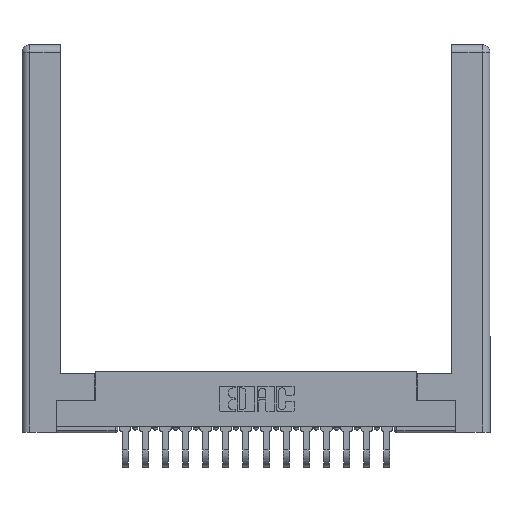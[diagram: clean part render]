
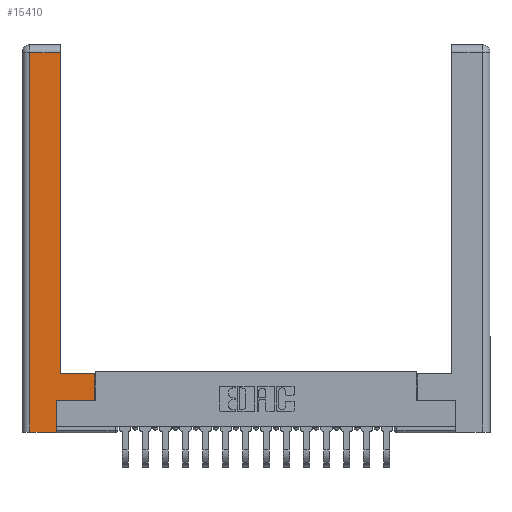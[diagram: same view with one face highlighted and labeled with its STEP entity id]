
A CAD part, top view. The second image highlights one B-rep face of the part: STEP entity #15410.
In plain terms, the highlighted planar face has unit normal (0, 0, 1).
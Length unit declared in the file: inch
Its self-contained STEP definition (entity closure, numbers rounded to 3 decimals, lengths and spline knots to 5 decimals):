
#453 = VECTOR ( 'NONE', #604, 39.37008 ) ;
#604 = DIRECTION ( 'NONE',  ( 0., 1., 0. ) ) ;
#621 = VERTEX_POINT ( 'NONE', #7658 ) ;
#630 = EDGE_CURVE ( 'NONE', #10348, #891, #4799, .T. ) ;
#891 = VERTEX_POINT ( 'NONE', #6131 ) ;
#920 = DIRECTION ( 'NONE',  ( -1., 0., 0. ) ) ;
#1051 = DIRECTION ( 'NONE',  ( 0., -1., 0. ) ) ;
#1247 = CARTESIAN_POINT ( 'NONE',  ( 0.295, 0.45, 0. ) ) ;
#1324 = ORIENTED_EDGE ( 'NONE', *, *, #15751, .T. ) ;
#2084 = DIRECTION ( 'NONE',  ( 0., 0., -1. ) ) ;
#2119 = DIRECTION ( 'NONE',  ( 0., 1., 0. ) ) ;
#2130 = DIRECTION ( 'NONE',  ( 0., 1., 0. ) ) ;
#2246 = ORIENTED_EDGE ( 'NONE', *, *, #14587, .T. ) ;
#2299 = LINE ( 'NONE', #14914, #3600 ) ;
#3600 = VECTOR ( 'NONE', #920, 39.37008 ) ;
#4054 = VERTEX_POINT ( 'NONE', #13711 ) ;
#4473 = LINE ( 'NONE', #1247, #9176 ) ;
#4799 = LINE ( 'NONE', #7370, #18181 ) ;
#4856 = CARTESIAN_POINT ( 'NONE',  ( 0., 0., 0. ) ) ;
#5283 = VECTOR ( 'NONE', #7096, 39.37008 ) ;
#5289 = EDGE_LOOP ( 'NONE', ( #7352, #12306, #13295, #8541, #2246, #16870, #6867, #1324 ) ) ;
#5706 = VERTEX_POINT ( 'NONE', #5848 ) ;
#5848 = CARTESIAN_POINT ( 'NONE',  ( 0.295, 0.45, 0. ) ) ;
#6032 = LINE ( 'NONE', #10174, #453 ) ;
#6131 = CARTESIAN_POINT ( 'NONE',  ( 0.565, 0.45, 0. ) ) ;
#6253 = AXIS2_PLACEMENT_3D ( 'NONE', #4856, #2084, #14791 ) ;
#6696 = DIRECTION ( 'NONE',  ( 1., 0., 0. ) ) ;
#6867 = ORIENTED_EDGE ( 'NONE', *, *, #630, .T. ) ;
#7035 = VECTOR ( 'NONE', #1051, 39.37008 ) ;
#7096 = DIRECTION ( 'NONE',  ( 1., 0., 0. ) ) ;
#7352 = ORIENTED_EDGE ( 'NONE', *, *, #12734, .T. ) ;
#7370 = CARTESIAN_POINT ( 'NONE',  ( 0.565, 0.45, 0. ) ) ;
#7658 = CARTESIAN_POINT ( 'NONE',  ( 0.265, 0.245, 0. ) ) ;
#7853 = CARTESIAN_POINT ( 'NONE',  ( 0.565, 0.245, 0. ) ) ;
#8409 = CARTESIAN_POINT ( 'NONE',  ( 0.0615, 0., 0. ) ) ;
#8541 = ORIENTED_EDGE ( 'NONE', *, *, #10479, .T. ) ;
#8675 = VERTEX_POINT ( 'NONE', #12777 ) ;
#8948 = LINE ( 'NONE', #14567, #13916 ) ;
#8949 = EDGE_CURVE ( 'NONE', #621, #10348, #16458, .T. ) ;
#9176 = VECTOR ( 'NONE', #18184, 39.37008 ) ;
#9451 = CARTESIAN_POINT ( 'NONE',  ( 0.295, 2.94, 0. ) ) ;
#9507 = VECTOR ( 'NONE', #6696, 39.37008 ) ;
#10174 = CARTESIAN_POINT ( 'NONE',  ( 0.295, 3., 0. ) ) ;
#10348 = VERTEX_POINT ( 'NONE', #7853 ) ;
#10479 = EDGE_CURVE ( 'NONE', #4054, #8675, #17044, .T. ) ;
#11164 = LINE ( 'NONE', #8409, #7035 ) ;
#11560 = CARTESIAN_POINT ( 'NONE',  ( 0.0615, 2.94, 0. ) ) ;
#11957 = EDGE_CURVE ( 'NONE', #16777, #12736, #2299, .T. ) ;
#12297 = CARTESIAN_POINT ( 'NONE',  ( 0.565, 0.245, 0. ) ) ;
#12306 = ORIENTED_EDGE ( 'NONE', *, *, #11957, .T. ) ;
#12734 = EDGE_CURVE ( 'NONE', #5706, #16777, #6032, .T. ) ;
#12736 = VERTEX_POINT ( 'NONE', #11560 ) ;
#12777 = CARTESIAN_POINT ( 'NONE',  ( 0.265, 0., 0. ) ) ;
#13295 = ORIENTED_EDGE ( 'NONE', *, *, #14189, .T. ) ;
#13711 = CARTESIAN_POINT ( 'NONE',  ( 0.0615, 0., 0. ) ) ;
#13916 = VECTOR ( 'NONE', #2130, 39.37008 ) ;
#13997 = CARTESIAN_POINT ( 'NONE',  ( 0.265, 0., 0. ) ) ;
#14189 = EDGE_CURVE ( 'NONE', #12736, #4054, #11164, .T. ) ;
#14520 = PLANE ( 'NONE',  #6253 ) ;
#14567 = CARTESIAN_POINT ( 'NONE',  ( 0.265, 0.245, 0. ) ) ;
#14587 = EDGE_CURVE ( 'NONE', #8675, #621, #8948, .T. ) ;
#14791 = DIRECTION ( 'NONE',  ( -1., 0., 0. ) ) ;
#14914 = CARTESIAN_POINT ( 'NONE',  ( 0.0615, 2.94, 0. ) ) ;
#15410 = ADVANCED_FACE ( 'NONE', ( #17464 ), #14520, .F. ) ;
#15751 = EDGE_CURVE ( 'NONE', #891, #5706, #4473, .T. ) ;
#16458 = LINE ( 'NONE', #12297, #9507 ) ;
#16777 = VERTEX_POINT ( 'NONE', #9451 ) ;
#16870 = ORIENTED_EDGE ( 'NONE', *, *, #8949, .T. ) ;
#17044 = LINE ( 'NONE', #13997, #5283 ) ;
#17464 = FACE_OUTER_BOUND ( 'NONE', #5289, .T. ) ;
#18181 = VECTOR ( 'NONE', #2119, 39.37008 ) ;
#18184 = DIRECTION ( 'NONE',  ( -1., 0., 0. ) ) ;
